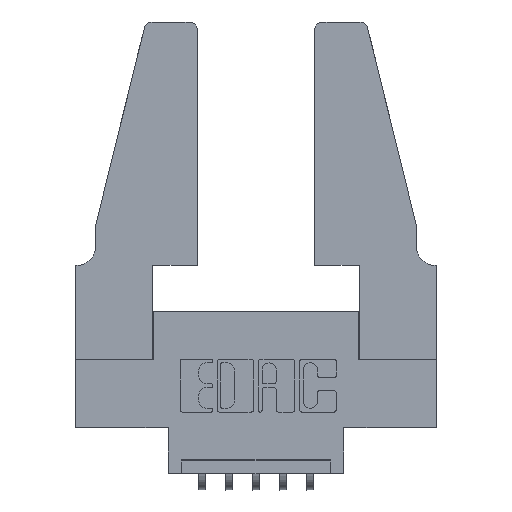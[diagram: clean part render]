
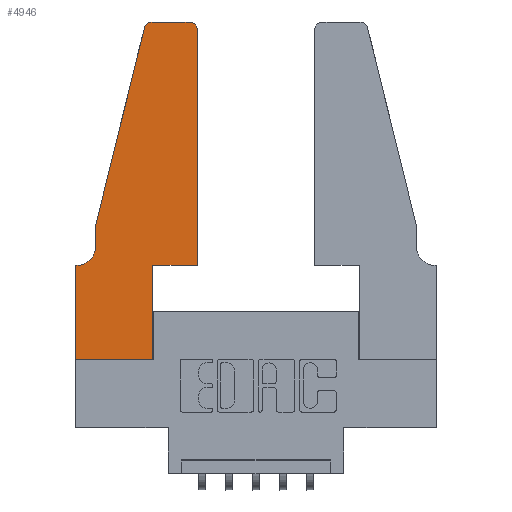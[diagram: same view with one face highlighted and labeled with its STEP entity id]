
A CAD part, top view. The second image highlights one B-rep face of the part: STEP entity #4946.
In plain terms, the highlighted planar face has unit normal (0, 0, 1).
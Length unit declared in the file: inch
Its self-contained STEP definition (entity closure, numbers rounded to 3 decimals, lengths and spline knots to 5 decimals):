
#113 = VERTEX_POINT ( 'NONE', #8729 ) ;
#150 = VERTEX_POINT ( 'NONE', #10309 ) ;
#178 = VECTOR ( 'NONE', #5826, 39.37008 ) ;
#223 = ORIENTED_EDGE ( 'NONE', *, *, #2866, .T. ) ;
#239 = DIRECTION ( 'NONE',  ( -1., 0., 0. ) ) ;
#298 = VERTEX_POINT ( 'NONE', #5389 ) ;
#386 = VERTEX_POINT ( 'NONE', #7097 ) ;
#570 = VERTEX_POINT ( 'NONE', #7469 ) ;
#621 = CIRCLE ( 'NONE', #9105, 0.03 ) ;
#692 = PLANE ( 'NONE',  #6377 ) ;
#778 = ORIENTED_EDGE ( 'NONE', *, *, #4287, .T. ) ;
#921 = CARTESIAN_POINT ( 'NONE',  ( 0., 0.35, 0.37 ) ) ;
#1293 = EDGE_CURVE ( 'NONE', #10121, #6495, #10614, .T. ) ;
#1360 = ORIENTED_EDGE ( 'NONE', *, *, #1293, .T. ) ;
#1478 = VECTOR ( 'NONE', #7551, 39.37008 ) ;
#1774 = VECTOR ( 'NONE', #6694, 39.37008 ) ;
#1780 = DIRECTION ( 'NONE',  ( 1., 0., 0. ) ) ;
#1822 = LINE ( 'NONE', #3379, #7868 ) ;
#1876 = DIRECTION ( 'NONE',  ( -1., 0., 0. ) ) ;
#2127 = LINE ( 'NONE', #5450, #3225 ) ;
#2220 = DIRECTION ( 'NONE',  ( 0., 0., -1. ) ) ;
#2267 = VERTEX_POINT ( 'NONE', #9301 ) ;
#2677 = CARTESIAN_POINT ( 'NONE',  ( 0.2865, 0., 0.37 ) ) ;
#2745 = ORIENTED_EDGE ( 'NONE', *, *, #8868, .T. ) ;
#2787 = CARTESIAN_POINT ( 'NONE',  ( 0.4505, 0.35, 0.37 ) ) ;
#2856 = EDGE_CURVE ( 'NONE', #386, #5063, #10700, .T. ) ;
#2866 = EDGE_CURVE ( 'NONE', #7538, #2267, #10963, .T. ) ;
#2957 = ORIENTED_EDGE ( 'NONE', *, *, #4880, .T. ) ;
#3225 = VECTOR ( 'NONE', #9874, 39.37008 ) ;
#3278 = VECTOR ( 'NONE', #239, 39.37008 ) ;
#3379 = CARTESIAN_POINT ( 'NONE',  ( 0.2605, 1.25, 0.37 ) ) ;
#3525 = DIRECTION ( 'NONE',  ( 1., 0., 0. ) ) ;
#3544 = DIRECTION ( 'NONE',  ( -0.239, -0.971, 0. ) ) ;
#3588 = LINE ( 'NONE', #5964, #178 ) ;
#3646 = LINE ( 'NONE', #4119, #1478 ) ;
#3783 = EDGE_CURVE ( 'NONE', #113, #570, #621, .T. ) ;
#3890 = VECTOR ( 'NONE', #6076, 39.37008 ) ;
#3947 = DIRECTION ( 'NONE',  ( 0., 1., 0. ) ) ;
#3971 = VERTEX_POINT ( 'NONE', #2677 ) ;
#4119 = CARTESIAN_POINT ( 'NONE',  ( 0., 0., 0.37 ) ) ;
#4121 = CARTESIAN_POINT ( 'NONE',  ( 0.4505, 0.35, 0.37 ) ) ;
#4208 = CARTESIAN_POINT ( 'NONE',  ( 0.0755, 0.42, 0.37 ) ) ;
#4237 = EDGE_LOOP ( 'NONE', ( #778, #2745, #223, #7774, #1360, #9716, #6943, #5935, #2957, #7104, #4892, #4756 ) ) ;
#4287 = EDGE_CURVE ( 'NONE', #570, #150, #1822, .T. ) ;
#4408 = CARTESIAN_POINT ( 'NONE',  ( 0.25487, 1.22718, 0.37 ) ) ;
#4413 = VECTOR ( 'NONE', #3544, 39.37008 ) ;
#4756 = ORIENTED_EDGE ( 'NONE', *, *, #3783, .T. ) ;
#4880 = EDGE_CURVE ( 'NONE', #3971, #298, #6786, .T. ) ;
#4892 = ORIENTED_EDGE ( 'NONE', *, *, #6123, .T. ) ;
#4905 = EDGE_CURVE ( 'NONE', #298, #7646, #3588, .T. ) ;
#4946 = ADVANCED_FACE ( 'NONE', ( #10017 ), #692, .T. ) ;
#5063 = VERTEX_POINT ( 'NONE', #7210 ) ;
#5389 = CARTESIAN_POINT ( 'NONE',  ( 0.2865, 0.35, 0.37 ) ) ;
#5450 = CARTESIAN_POINT ( 'NONE',  ( 0.0755, 0.5, 0.37 ) ) ;
#5826 = DIRECTION ( 'NONE',  ( 1., 0., 0. ) ) ;
#5935 = ORIENTED_EDGE ( 'NONE', *, *, #9240, .T. ) ;
#5964 = CARTESIAN_POINT ( 'NONE',  ( 0.4505, 0.35, 0.37 ) ) ;
#6057 = CARTESIAN_POINT ( 'NONE',  ( 0.4205, 1.22, 0.37 ) ) ;
#6076 = DIRECTION ( 'NONE',  ( 0., -1., 0. ) ) ;
#6123 = EDGE_CURVE ( 'NONE', #7646, #113, #6625, .T. ) ;
#6377 = AXIS2_PLACEMENT_3D ( 'NONE', #921, #6964, #1780 ) ;
#6378 = EDGE_CURVE ( 'NONE', #6495, #386, #7146, .T. ) ;
#6495 = VERTEX_POINT ( 'NONE', #10683 ) ;
#6625 = LINE ( 'NONE', #4121, #1774 ) ;
#6694 = DIRECTION ( 'NONE',  ( 0., 1., 0. ) ) ;
#6786 = LINE ( 'NONE', #9373, #10542 ) ;
#6943 = ORIENTED_EDGE ( 'NONE', *, *, #2856, .T. ) ;
#6964 = DIRECTION ( 'NONE',  ( 0., 0., 1. ) ) ;
#7097 = CARTESIAN_POINT ( 'NONE',  ( 0., 0.35, 0.37 ) ) ;
#7104 = ORIENTED_EDGE ( 'NONE', *, *, #4905, .T. ) ;
#7146 = LINE ( 'NONE', #9617, #3278 ) ;
#7210 = CARTESIAN_POINT ( 'NONE',  ( 0., 0., 0.37 ) ) ;
#7469 = CARTESIAN_POINT ( 'NONE',  ( 0.4205, 1.25, 0.37 ) ) ;
#7538 = VERTEX_POINT ( 'NONE', #4408 ) ;
#7551 = DIRECTION ( 'NONE',  ( 1., 0., 0. ) ) ;
#7569 = AXIS2_PLACEMENT_3D ( 'NONE', #9820, #2220, #9891 ) ;
#7646 = VERTEX_POINT ( 'NONE', #2787 ) ;
#7774 = ORIENTED_EDGE ( 'NONE', *, *, #9753, .T. ) ;
#7868 = VECTOR ( 'NONE', #1876, 39.37008 ) ;
#8636 = DIRECTION ( 'NONE',  ( 0., 0., 1. ) ) ;
#8729 = CARTESIAN_POINT ( 'NONE',  ( 0.4505, 1.22, 0.37 ) ) ;
#8868 = EDGE_CURVE ( 'NONE', #150, #7538, #10213, .T. ) ;
#9105 = AXIS2_PLACEMENT_3D ( 'NONE', #6057, #8636, #3525 ) ;
#9240 = EDGE_CURVE ( 'NONE', #5063, #3971, #3646, .T. ) ;
#9301 = CARTESIAN_POINT ( 'NONE',  ( 0.0755, 0.5, 0.37 ) ) ;
#9373 = CARTESIAN_POINT ( 'NONE',  ( 0.2865, 0.35, 0.37 ) ) ;
#9489 = CARTESIAN_POINT ( 'NONE',  ( 0.0755, 0.5, 0.37 ) ) ;
#9561 = CARTESIAN_POINT ( 'NONE',  ( 0.284, 1.22, 0.37 ) ) ;
#9617 = CARTESIAN_POINT ( 'NONE',  ( 0.0755, 0.35, 0.37 ) ) ;
#9716 = ORIENTED_EDGE ( 'NONE', *, *, #6378, .T. ) ;
#9753 = EDGE_CURVE ( 'NONE', #2267, #10121, #2127, .T. ) ;
#9820 = CARTESIAN_POINT ( 'NONE',  ( 0.0055, 0.42, 0.37 ) ) ;
#9874 = DIRECTION ( 'NONE',  ( 0., -1., 0. ) ) ;
#9891 = DIRECTION ( 'NONE',  ( -1., 0., 0. ) ) ;
#10017 = FACE_OUTER_BOUND ( 'NONE', #4237, .T. ) ;
#10121 = VERTEX_POINT ( 'NONE', #4208 ) ;
#10213 = CIRCLE ( 'NONE', #10365, 0.03 ) ;
#10309 = CARTESIAN_POINT ( 'NONE',  ( 0.284, 1.25, 0.37 ) ) ;
#10310 = DIRECTION ( 'NONE',  ( 0., 0., 1. ) ) ;
#10358 = CARTESIAN_POINT ( 'NONE',  ( 0., 0., 0.37 ) ) ;
#10365 = AXIS2_PLACEMENT_3D ( 'NONE', #9561, #10310, #10419 ) ;
#10419 = DIRECTION ( 'NONE',  ( 1., 0., 0. ) ) ;
#10542 = VECTOR ( 'NONE', #3947, 39.37008 ) ;
#10614 = CIRCLE ( 'NONE', #7569, 0.07 ) ;
#10683 = CARTESIAN_POINT ( 'NONE',  ( 0.0055, 0.35, 0.37 ) ) ;
#10700 = LINE ( 'NONE', #10358, #3890 ) ;
#10963 = LINE ( 'NONE', #9489, #4413 ) ;
